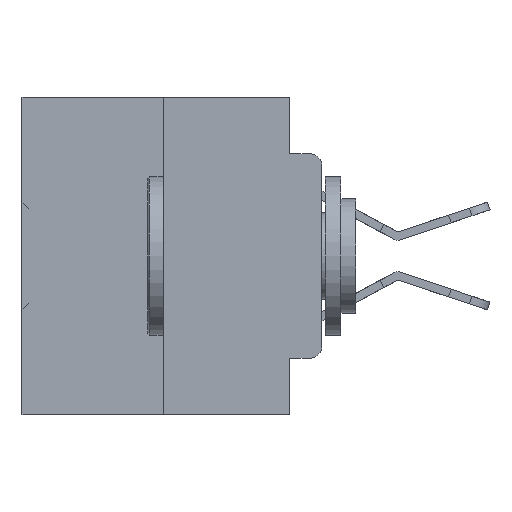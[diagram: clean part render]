
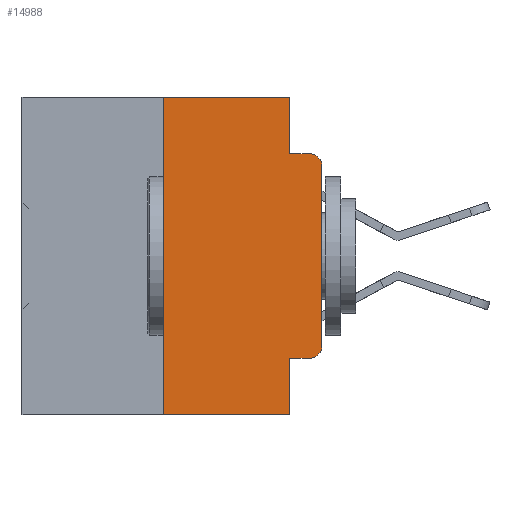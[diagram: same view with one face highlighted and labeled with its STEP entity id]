
A CAD part, left-side view. The second image highlights one B-rep face of the part: STEP entity #14988.
In plain terms, the highlighted planar face has unit normal (-1, 0, 0).
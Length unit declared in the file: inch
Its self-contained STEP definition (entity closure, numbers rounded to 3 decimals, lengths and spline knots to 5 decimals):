
#87 = ORIENTED_EDGE ( 'NONE', *, *, #26849, .T. ) ;
#103 = VERTEX_POINT ( 'NONE', #24795 ) ;
#812 = DIRECTION ( 'NONE',  ( 0., 0., -1. ) ) ;
#820 = CARTESIAN_POINT ( 'NONE',  ( 0., 0.02, -0.4115 ) ) ;
#899 = DIRECTION ( 'NONE',  ( -1., 0., 0. ) ) ;
#1185 = VERTEX_POINT ( 'NONE', #9882 ) ;
#1343 = CARTESIAN_POINT ( 'NONE',  ( 0., 0.473, -0.5 ) ) ;
#1868 = DIRECTION ( 'NONE',  ( 1., 0., 0. ) ) ;
#2787 = VECTOR ( 'NONE', #14065, 39.37008 ) ;
#3515 = ORIENTED_EDGE ( 'NONE', *, *, #10278, .T. ) ;
#4380 = DIRECTION ( 'NONE',  ( 0., -1., 0. ) ) ;
#4451 = LINE ( 'NONE', #20270, #9645 ) ;
#4527 = CARTESIAN_POINT ( 'NONE',  ( 0., 0.051, -0.0885 ) ) ;
#6030 = CARTESIAN_POINT ( 'NONE',  ( 0., 0.25, -0.5 ) ) ;
#6150 = CIRCLE ( 'NONE', #7059, 0.02 ) ;
#6291 = CARTESIAN_POINT ( 'NONE',  ( 0., 0., -0.1085 ) ) ;
#7010 = VECTOR ( 'NONE', #16023, 39.37008 ) ;
#7059 = AXIS2_PLACEMENT_3D ( 'NONE', #34424, #19413, #812 ) ;
#7225 = VERTEX_POINT ( 'NONE', #820 ) ;
#7261 = FACE_OUTER_BOUND ( 'NONE', #9818, .T. ) ;
#7272 = CARTESIAN_POINT ( 'NONE',  ( 0., 0.051, -0.0885 ) ) ;
#8046 = ORIENTED_EDGE ( 'NONE', *, *, #26989, .T. ) ;
#8375 = CARTESIAN_POINT ( 'NONE',  ( 0., 0.473, 0. ) ) ;
#8692 = VECTOR ( 'NONE', #13737, 39.37008 ) ;
#9329 = ORIENTED_EDGE ( 'NONE', *, *, #35034, .F. ) ;
#9456 = VECTOR ( 'NONE', #28216, 39.37008 ) ;
#9645 = VECTOR ( 'NONE', #10675, 39.37008 ) ;
#9818 = EDGE_LOOP ( 'NONE', ( #8046, #3515, #20959, #37284, #26288, #10284, #87, #9329, #35181, #26096 ) ) ;
#9882 = CARTESIAN_POINT ( 'NONE',  ( 0., 0.051, -0.4115 ) ) ;
#10278 = EDGE_CURVE ( 'NONE', #16433, #32718, #6150, .T. ) ;
#10284 = ORIENTED_EDGE ( 'NONE', *, *, #35775, .F. ) ;
#10471 = AXIS2_PLACEMENT_3D ( 'NONE', #8375, #1868, #29155 ) ;
#10675 = DIRECTION ( 'NONE',  ( 0., 0., -1. ) ) ;
#10786 = EDGE_CURVE ( 'NONE', #103, #10993, #22125, .T. ) ;
#10993 = VERTEX_POINT ( 'NONE', #13480 ) ;
#11277 = CARTESIAN_POINT ( 'NONE',  ( 0., 0., 0. ) ) ;
#11391 = PLANE ( 'NONE',  #10471 ) ;
#12342 = VECTOR ( 'NONE', #34778, 39.37008 ) ;
#13480 = CARTESIAN_POINT ( 'NONE',  ( 0., 0.051, 0. ) ) ;
#13522 = EDGE_CURVE ( 'NONE', #1185, #7225, #33153, .T. ) ;
#13737 = DIRECTION ( 'NONE',  ( 0., -1., 0. ) ) ;
#14065 = DIRECTION ( 'NONE',  ( 0., 0., 1. ) ) ;
#14164 = VECTOR ( 'NONE', #4380, 39.37008 ) ;
#14934 = EDGE_CURVE ( 'NONE', #7225, #23886, #17181, .T. ) ;
#14988 = ADVANCED_FACE ( 'NONE', ( #7261 ), #11391, .F. ) ;
#15763 = CARTESIAN_POINT ( 'NONE',  ( 0., 0.051, 0. ) ) ;
#16023 = DIRECTION ( 'NONE',  ( 0., 0., -1. ) ) ;
#16433 = VERTEX_POINT ( 'NONE', #6291 ) ;
#16936 = LINE ( 'NONE', #15763, #7010 ) ;
#17043 = VERTEX_POINT ( 'NONE', #34443 ) ;
#17158 = VECTOR ( 'NONE', #32453, 39.37008 ) ;
#17181 = CIRCLE ( 'NONE', #33178, 0.02 ) ;
#17654 = VERTEX_POINT ( 'NONE', #4527 ) ;
#18996 = CARTESIAN_POINT ( 'NONE',  ( 0., 0.473, 0. ) ) ;
#19413 = DIRECTION ( 'NONE',  ( -1., 0., 0. ) ) ;
#20270 = CARTESIAN_POINT ( 'NONE',  ( 0., 0.051, 0. ) ) ;
#20346 = CARTESIAN_POINT ( 'NONE',  ( 0., 0.25, 0. ) ) ;
#20487 = EDGE_CURVE ( 'NONE', #10993, #17654, #16936, .T. ) ;
#20959 = ORIENTED_EDGE ( 'NONE', *, *, #31758, .F. ) ;
#22007 = DIRECTION ( 'NONE',  ( 0., 0., -1. ) ) ;
#22125 = LINE ( 'NONE', #18996, #9456 ) ;
#22590 = LINE ( 'NONE', #11277, #2787 ) ;
#23886 = VERTEX_POINT ( 'NONE', #33042 ) ;
#24795 = CARTESIAN_POINT ( 'NONE',  ( 0., 0.25, 0. ) ) ;
#25547 = CARTESIAN_POINT ( 'NONE',  ( 0., 0.051, -0.4115 ) ) ;
#26096 = ORIENTED_EDGE ( 'NONE', *, *, #14934, .T. ) ;
#26288 = ORIENTED_EDGE ( 'NONE', *, *, #10786, .F. ) ;
#26849 = EDGE_CURVE ( 'NONE', #32638, #17043, #32526, .T. ) ;
#26989 = EDGE_CURVE ( 'NONE', #23886, #16433, #22590, .T. ) ;
#28216 = DIRECTION ( 'NONE',  ( 0., -1., 0. ) ) ;
#29155 = DIRECTION ( 'NONE',  ( 0., 0., -1. ) ) ;
#31758 = EDGE_CURVE ( 'NONE', #17654, #32718, #34484, .T. ) ;
#32453 = DIRECTION ( 'NONE',  ( 0., 0., 1. ) ) ;
#32526 = LINE ( 'NONE', #1343, #14164 ) ;
#32638 = VERTEX_POINT ( 'NONE', #6030 ) ;
#32718 = VERTEX_POINT ( 'NONE', #33501 ) ;
#33042 = CARTESIAN_POINT ( 'NONE',  ( 0., 0., -0.3915 ) ) ;
#33153 = LINE ( 'NONE', #25547, #8692 ) ;
#33178 = AXIS2_PLACEMENT_3D ( 'NONE', #33987, #899, #22007 ) ;
#33501 = CARTESIAN_POINT ( 'NONE',  ( 0., 0.02, -0.0885 ) ) ;
#33987 = CARTESIAN_POINT ( 'NONE',  ( 0., 0.02, -0.3915 ) ) ;
#34424 = CARTESIAN_POINT ( 'NONE',  ( 0., 0.02, -0.1085 ) ) ;
#34443 = CARTESIAN_POINT ( 'NONE',  ( 0., 0.051, -0.5 ) ) ;
#34484 = LINE ( 'NONE', #7272, #12342 ) ;
#34778 = DIRECTION ( 'NONE',  ( 0., -1., 0. ) ) ;
#35034 = EDGE_CURVE ( 'NONE', #1185, #17043, #4451, .T. ) ;
#35181 = ORIENTED_EDGE ( 'NONE', *, *, #13522, .T. ) ;
#35775 = EDGE_CURVE ( 'NONE', #32638, #103, #35925, .T. ) ;
#35925 = LINE ( 'NONE', #20346, #17158 ) ;
#37284 = ORIENTED_EDGE ( 'NONE', *, *, #20487, .F. ) ;
